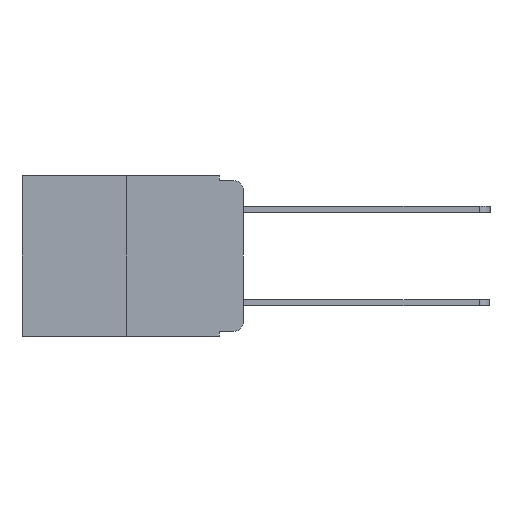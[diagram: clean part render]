
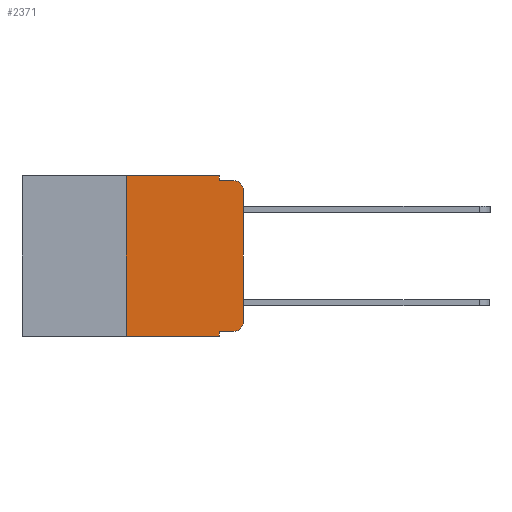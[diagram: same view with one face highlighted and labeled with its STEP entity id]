
A CAD part, left-side view. The second image highlights one B-rep face of the part: STEP entity #2371.
In plain terms, the highlighted planar face has unit normal (-1, 0, 0).
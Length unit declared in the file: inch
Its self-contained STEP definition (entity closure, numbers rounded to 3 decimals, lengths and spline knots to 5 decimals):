
#57 = DIRECTION ( 'NONE',  ( 0., 0., -1. ) ) ;
#478 = DIRECTION ( 'NONE',  ( 0., 0., -1. ) ) ;
#602 = ORIENTED_EDGE ( 'NONE', *, *, #2896, .T. ) ;
#729 = CARTESIAN_POINT ( 'NONE',  ( 0., 0.473, 0. ) ) ;
#730 = CIRCLE ( 'NONE', #9793, 0.02 ) ;
#753 = VECTOR ( 'NONE', #478, 39.37008 ) ;
#896 = LINE ( 'NONE', #6922, #5783 ) ;
#1295 = VERTEX_POINT ( 'NONE', #6171 ) ;
#1368 = DIRECTION ( 'NONE',  ( 0., 0., -1. ) ) ;
#1460 = VERTEX_POINT ( 'NONE', #2138 ) ;
#1573 = CARTESIAN_POINT ( 'NONE',  ( 0., 0.02, -0.333 ) ) ;
#1816 = LINE ( 'NONE', #7328, #10610 ) ;
#1836 = CARTESIAN_POINT ( 'NONE',  ( 0., 0.051, -0.01 ) ) ;
#1854 = DIRECTION ( 'NONE',  ( 0., -1., 0. ) ) ;
#1944 = DIRECTION ( 'NONE',  ( 0., -1., 0. ) ) ;
#2138 = CARTESIAN_POINT ( 'NONE',  ( 0., 0.051, -0.333 ) ) ;
#2164 = EDGE_CURVE ( 'NONE', #6990, #10501, #730, .T. ) ;
#2175 = VERTEX_POINT ( 'NONE', #7814 ) ;
#2187 = VERTEX_POINT ( 'NONE', #10973 ) ;
#2371 = ADVANCED_FACE ( 'NONE', ( #9594 ), #7576, .F. ) ;
#2651 = CARTESIAN_POINT ( 'NONE',  ( 0., 0.02, -0.313 ) ) ;
#2896 = EDGE_CURVE ( 'NONE', #1460, #6990, #6754, .T. ) ;
#3058 = DIRECTION ( 'NONE',  ( 0., 0., 1. ) ) ;
#3246 = DIRECTION ( 'NONE',  ( 0., 0., 1. ) ) ;
#3542 = EDGE_CURVE ( 'NONE', #1460, #2187, #10407, .T. ) ;
#3626 = DIRECTION ( 'NONE',  ( 0., 0., -1. ) ) ;
#4112 = EDGE_CURVE ( 'NONE', #8173, #6899, #6954, .T. ) ;
#4156 = CARTESIAN_POINT ( 'NONE',  ( 0., 0., 0. ) ) ;
#4181 = EDGE_CURVE ( 'NONE', #5377, #8173, #1816, .T. ) ;
#4216 = CARTESIAN_POINT ( 'NONE',  ( 0., 0.02, -0.01 ) ) ;
#4450 = CIRCLE ( 'NONE', #9750, 0.02 ) ;
#4504 = CARTESIAN_POINT ( 'NONE',  ( 0., 0.051, 0. ) ) ;
#4588 = CARTESIAN_POINT ( 'NONE',  ( 0., 0.051, 0. ) ) ;
#4726 = EDGE_CURVE ( 'NONE', #6899, #2175, #896, .T. ) ;
#4824 = DIRECTION ( 'NONE',  ( 0., -1., 0. ) ) ;
#4844 = CARTESIAN_POINT ( 'NONE',  ( 0., 0.25, -0.343 ) ) ;
#4917 = ORIENTED_EDGE ( 'NONE', *, *, #6445, .T. ) ;
#4941 = ORIENTED_EDGE ( 'NONE', *, *, #4726, .F. ) ;
#5134 = EDGE_LOOP ( 'NONE', ( #4917, #8944, #8680, #4941, #8665, #5542, #7710, #6869, #602, #11007 ) ) ;
#5192 = DIRECTION ( 'NONE',  ( -1., 0., 0. ) ) ;
#5232 = LINE ( 'NONE', #8781, #11055 ) ;
#5315 = EDGE_CURVE ( 'NONE', #2175, #6530, #11169, .T. ) ;
#5377 = VERTEX_POINT ( 'NONE', #4844 ) ;
#5542 = ORIENTED_EDGE ( 'NONE', *, *, #4181, .F. ) ;
#5783 = VECTOR ( 'NONE', #1368, 39.37008 ) ;
#5879 = EDGE_CURVE ( 'NONE', #1295, #6530, #4450, .T. ) ;
#5996 = DIRECTION ( 'NONE',  ( 1., 0., 0. ) ) ;
#6171 = CARTESIAN_POINT ( 'NONE',  ( 0., 0., -0.03 ) ) ;
#6247 = VECTOR ( 'NONE', #1944, 39.37008 ) ;
#6351 = CARTESIAN_POINT ( 'NONE',  ( 0., 0.25, 0. ) ) ;
#6445 = EDGE_CURVE ( 'NONE', #10501, #1295, #10359, .T. ) ;
#6530 = VERTEX_POINT ( 'NONE', #4216 ) ;
#6754 = LINE ( 'NONE', #7309, #6247 ) ;
#6869 = ORIENTED_EDGE ( 'NONE', *, *, #3542, .F. ) ;
#6899 = VERTEX_POINT ( 'NONE', #4504 ) ;
#6922 = CARTESIAN_POINT ( 'NONE',  ( 0., 0.051, 0. ) ) ;
#6954 = LINE ( 'NONE', #729, #8778 ) ;
#6990 = VERTEX_POINT ( 'NONE', #1573 ) ;
#7064 = VECTOR ( 'NONE', #11140, 39.37008 ) ;
#7308 = EDGE_CURVE ( 'NONE', #5377, #2187, #5232, .T. ) ;
#7309 = CARTESIAN_POINT ( 'NONE',  ( 0., 0.051, -0.333 ) ) ;
#7328 = CARTESIAN_POINT ( 'NONE',  ( 0., 0.25, 0. ) ) ;
#7549 = CARTESIAN_POINT ( 'NONE',  ( 0., 0.473, 0. ) ) ;
#7576 = PLANE ( 'NONE',  #9403 ) ;
#7710 = ORIENTED_EDGE ( 'NONE', *, *, #7308, .T. ) ;
#7814 = CARTESIAN_POINT ( 'NONE',  ( 0., 0.051, -0.01 ) ) ;
#8173 = VERTEX_POINT ( 'NONE', #6351 ) ;
#8265 = VECTOR ( 'NONE', #3246, 39.37008 ) ;
#8591 = DIRECTION ( 'NONE',  ( -1., 0., 0. ) ) ;
#8665 = ORIENTED_EDGE ( 'NONE', *, *, #4112, .F. ) ;
#8680 = ORIENTED_EDGE ( 'NONE', *, *, #5315, .F. ) ;
#8778 = VECTOR ( 'NONE', #4824, 39.37008 ) ;
#8781 = CARTESIAN_POINT ( 'NONE',  ( 0., 0.473, -0.343 ) ) ;
#8944 = ORIENTED_EDGE ( 'NONE', *, *, #5879, .T. ) ;
#9150 = CARTESIAN_POINT ( 'NONE',  ( 0., 0., -0.313 ) ) ;
#9403 = AXIS2_PLACEMENT_3D ( 'NONE', #7549, #5996, #57 ) ;
#9594 = FACE_OUTER_BOUND ( 'NONE', #5134, .T. ) ;
#9750 = AXIS2_PLACEMENT_3D ( 'NONE', #9984, #5192, #10745 ) ;
#9793 = AXIS2_PLACEMENT_3D ( 'NONE', #2651, #8591, #3626 ) ;
#9984 = CARTESIAN_POINT ( 'NONE',  ( 0., 0.02, -0.03 ) ) ;
#10359 = LINE ( 'NONE', #4156, #8265 ) ;
#10407 = LINE ( 'NONE', #4588, #753 ) ;
#10501 = VERTEX_POINT ( 'NONE', #9150 ) ;
#10610 = VECTOR ( 'NONE', #3058, 39.37008 ) ;
#10745 = DIRECTION ( 'NONE',  ( 0., 0., -1. ) ) ;
#10973 = CARTESIAN_POINT ( 'NONE',  ( 0., 0.051, -0.343 ) ) ;
#11007 = ORIENTED_EDGE ( 'NONE', *, *, #2164, .T. ) ;
#11055 = VECTOR ( 'NONE', #1854, 39.37008 ) ;
#11140 = DIRECTION ( 'NONE',  ( 0., -1., 0. ) ) ;
#11169 = LINE ( 'NONE', #1836, #7064 ) ;
